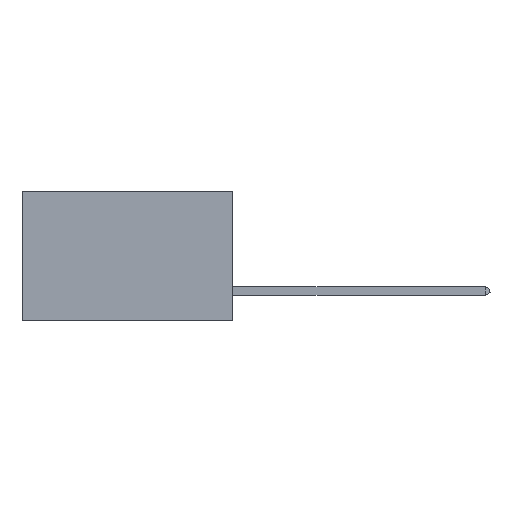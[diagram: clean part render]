
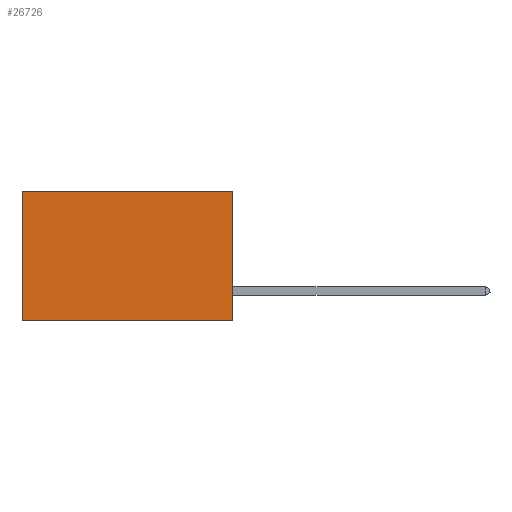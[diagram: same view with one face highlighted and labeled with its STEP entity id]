
A CAD part, left-side view. The second image highlights one B-rep face of the part: STEP entity #26726.
In plain terms, the highlighted planar face has unit normal (-1, 0, 0).
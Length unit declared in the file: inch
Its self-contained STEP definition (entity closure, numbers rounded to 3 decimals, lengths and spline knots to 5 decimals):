
#912 = EDGE_CURVE ( 'NONE', #15389, #24501, #6209, .T. ) ;
#1386 = LINE ( 'NONE', #17745, #34253 ) ;
#1671 = AXIS2_PLACEMENT_3D ( 'NONE', #16752, #13953, #19408 ) ;
#2427 = VERTEX_POINT ( 'NONE', #20575 ) ;
#4350 = LINE ( 'NONE', #23167, #18507 ) ;
#4956 = CARTESIAN_POINT ( 'NONE',  ( 0.2875, 0.6, -0.37 ) ) ;
#6209 = LINE ( 'NONE', #29589, #29517 ) ;
#7019 = DIRECTION ( 'NONE',  ( 0., 1., 0. ) ) ;
#7479 = ORIENTED_EDGE ( 'NONE', *, *, #25964, .T. ) ;
#8173 = DIRECTION ( 'NONE',  ( 0., 0., -1. ) ) ;
#10140 = ORIENTED_EDGE ( 'NONE', *, *, #18621, .F. ) ;
#10323 = EDGE_CURVE ( 'NONE', #2427, #24501, #1386, .T. ) ;
#11246 = PLANE ( 'NONE',  #1671 ) ;
#12117 = DIRECTION ( 'NONE',  ( 0., 1., 0. ) ) ;
#13953 = DIRECTION ( 'NONE',  ( 1., 0., 0. ) ) ;
#15217 = VERTEX_POINT ( 'NONE', #19287 ) ;
#15389 = VERTEX_POINT ( 'NONE', #34164 ) ;
#16752 = CARTESIAN_POINT ( 'NONE',  ( 0.2875, 0., 0. ) ) ;
#17680 = VECTOR ( 'NONE', #31970, 39.37008 ) ;
#17745 = CARTESIAN_POINT ( 'NONE',  ( 0.2875, 0., -0.37 ) ) ;
#18340 = EDGE_LOOP ( 'NONE', ( #27297, #31754, #10140, #7479 ) ) ;
#18507 = VECTOR ( 'NONE', #7019, 39.37008 ) ;
#18621 = EDGE_CURVE ( 'NONE', #15217, #2427, #25162, .T. ) ;
#19287 = CARTESIAN_POINT ( 'NONE',  ( 0.2875, 0., 0. ) ) ;
#19408 = DIRECTION ( 'NONE',  ( 0., 0., -1. ) ) ;
#20575 = CARTESIAN_POINT ( 'NONE',  ( 0.2875, 0., -0.37 ) ) ;
#23167 = CARTESIAN_POINT ( 'NONE',  ( 0.2875, 0., 0. ) ) ;
#24501 = VERTEX_POINT ( 'NONE', #4956 ) ;
#25162 = LINE ( 'NONE', #27311, #17680 ) ;
#25964 = EDGE_CURVE ( 'NONE', #15217, #15389, #4350, .T. ) ;
#26726 = ADVANCED_FACE ( 'NONE', ( #29292 ), #11246, .F. ) ;
#27297 = ORIENTED_EDGE ( 'NONE', *, *, #912, .T. ) ;
#27311 = CARTESIAN_POINT ( 'NONE',  ( 0.2875, 0., 0. ) ) ;
#29292 = FACE_OUTER_BOUND ( 'NONE', #18340, .T. ) ;
#29517 = VECTOR ( 'NONE', #8173, 39.37008 ) ;
#29589 = CARTESIAN_POINT ( 'NONE',  ( 0.2875, 0.6, 0. ) ) ;
#31754 = ORIENTED_EDGE ( 'NONE', *, *, #10323, .F. ) ;
#31970 = DIRECTION ( 'NONE',  ( 0., 0., -1. ) ) ;
#34164 = CARTESIAN_POINT ( 'NONE',  ( 0.2875, 0.6, 0. ) ) ;
#34253 = VECTOR ( 'NONE', #12117, 39.37008 ) ;
